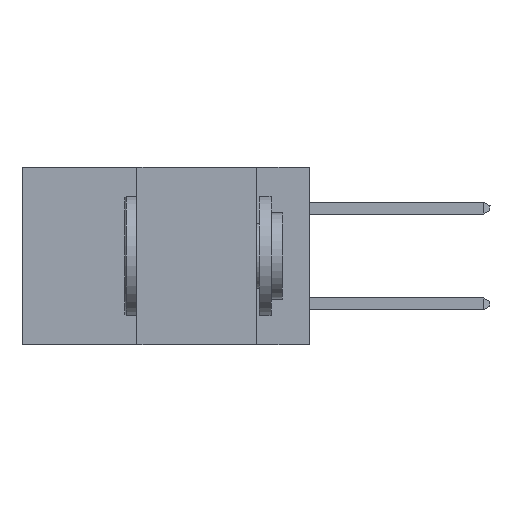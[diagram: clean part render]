
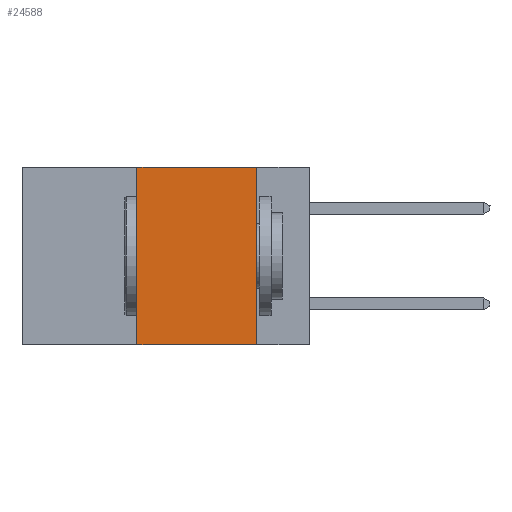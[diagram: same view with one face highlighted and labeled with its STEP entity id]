
A CAD part, left-side view. The second image highlights one B-rep face of the part: STEP entity #24588.
In plain terms, the highlighted planar face has unit normal (-1, 0, 0).
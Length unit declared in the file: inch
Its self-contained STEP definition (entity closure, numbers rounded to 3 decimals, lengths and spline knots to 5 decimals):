
#1562 = CARTESIAN_POINT ( 'NONE',  ( 0., 0.6, 0. ) ) ;
#1738 = VECTOR ( 'NONE', #2532, 39.37008 ) ;
#2532 = DIRECTION ( 'NONE',  ( 0., 0., -1. ) ) ;
#3132 = PLANE ( 'NONE',  #8682 ) ;
#4058 = EDGE_CURVE ( 'NONE', #20268, #15881, #22576, .T. ) ;
#5996 = VERTEX_POINT ( 'NONE', #23018 ) ;
#7552 = LINE ( 'NONE', #23243, #8776 ) ;
#8083 = CARTESIAN_POINT ( 'NONE',  ( 0., 0.6, 0. ) ) ;
#8682 = AXIS2_PLACEMENT_3D ( 'NONE', #1562, #25070, #19303 ) ;
#8776 = VECTOR ( 'NONE', #9837, 39.37008 ) ;
#8802 = ORIENTED_EDGE ( 'NONE', *, *, #4058, .F. ) ;
#8860 = EDGE_LOOP ( 'NONE', ( #19809, #8802, #19935, #18481 ) ) ;
#9044 = LINE ( 'NONE', #18439, #23116 ) ;
#9577 = CARTESIAN_POINT ( 'NONE',  ( 0., 0.11, 0. ) ) ;
#9837 = DIRECTION ( 'NONE',  ( 0., -1., 0. ) ) ;
#10701 = EDGE_CURVE ( 'NONE', #11587, #5996, #7552, .T. ) ;
#11587 = VERTEX_POINT ( 'NONE', #18513 ) ;
#15544 = EDGE_CURVE ( 'NONE', #15881, #5996, #20734, .T. ) ;
#15881 = VERTEX_POINT ( 'NONE', #9577 ) ;
#16754 = VECTOR ( 'NONE', #17812, 39.37008 ) ;
#17812 = DIRECTION ( 'NONE',  ( 0., -1., 0. ) ) ;
#18133 = CARTESIAN_POINT ( 'NONE',  ( 0., 0.11, 0. ) ) ;
#18439 = CARTESIAN_POINT ( 'NONE',  ( 0., 0.36, 0. ) ) ;
#18481 = ORIENTED_EDGE ( 'NONE', *, *, #10701, .T. ) ;
#18513 = CARTESIAN_POINT ( 'NONE',  ( 0., 0.36, -0.37 ) ) ;
#19303 = DIRECTION ( 'NONE',  ( 0., 0., -1. ) ) ;
#19809 = ORIENTED_EDGE ( 'NONE', *, *, #15544, .F. ) ;
#19935 = ORIENTED_EDGE ( 'NONE', *, *, #24856, .F. ) ;
#20268 = VERTEX_POINT ( 'NONE', #20910 ) ;
#20385 = DIRECTION ( 'NONE',  ( 0., 0., 1. ) ) ;
#20734 = LINE ( 'NONE', #18133, #1738 ) ;
#20910 = CARTESIAN_POINT ( 'NONE',  ( 0., 0.36, 0. ) ) ;
#21282 = FACE_OUTER_BOUND ( 'NONE', #8860, .T. ) ;
#22576 = LINE ( 'NONE', #8083, #16754 ) ;
#23018 = CARTESIAN_POINT ( 'NONE',  ( 0., 0.11, -0.37 ) ) ;
#23116 = VECTOR ( 'NONE', #20385, 39.37008 ) ;
#23243 = CARTESIAN_POINT ( 'NONE',  ( 0., 0.6, -0.37 ) ) ;
#24588 = ADVANCED_FACE ( 'NONE', ( #21282 ), #3132, .F. ) ;
#24856 = EDGE_CURVE ( 'NONE', #11587, #20268, #9044, .T. ) ;
#25070 = DIRECTION ( 'NONE',  ( 1., 0., 0. ) ) ;
